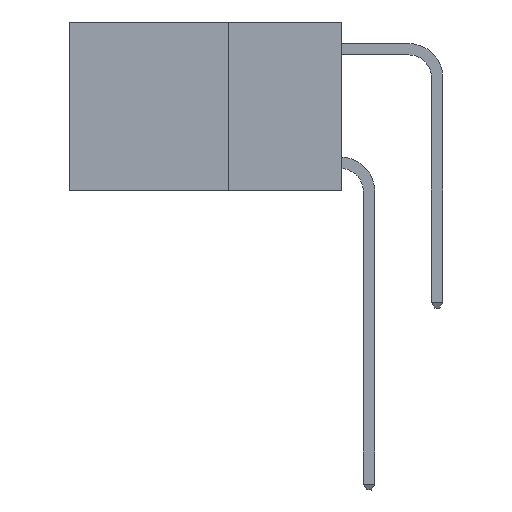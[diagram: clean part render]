
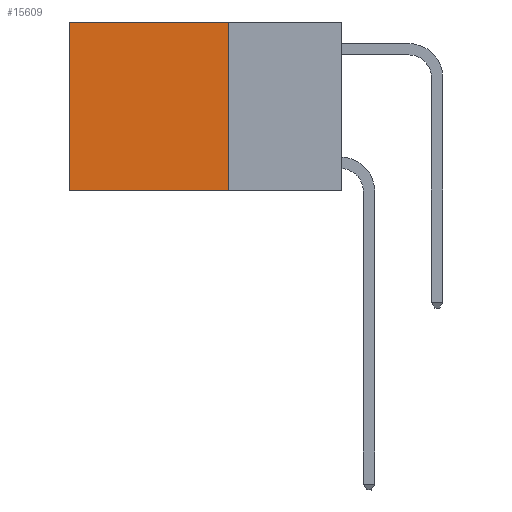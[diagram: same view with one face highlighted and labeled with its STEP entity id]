
A CAD part, left-side view. The second image highlights one B-rep face of the part: STEP entity #15609.
In plain terms, the highlighted planar face has unit normal (-1, 0, 0).
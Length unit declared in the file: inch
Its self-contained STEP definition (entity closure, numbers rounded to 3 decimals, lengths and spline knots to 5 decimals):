
#139 = DIRECTION ( 'NONE',  ( 0., 0., -1. ) ) ;
#140 = VERTEX_POINT ( 'NONE', #27110 ) ;
#480 = CARTESIAN_POINT ( 'NONE',  ( 0.2625, 0.25, -0.37 ) ) ;
#797 = LINE ( 'NONE', #14445, #27979 ) ;
#2272 = VERTEX_POINT ( 'NONE', #8109 ) ;
#2958 = ORIENTED_EDGE ( 'NONE', *, *, #20229, .F. ) ;
#4125 = CARTESIAN_POINT ( 'NONE',  ( 0.2625, 0.25, 0. ) ) ;
#4859 = DIRECTION ( 'NONE',  ( 1., 0., 0. ) ) ;
#5541 = ORIENTED_EDGE ( 'NONE', *, *, #27164, .T. ) ;
#6876 = CARTESIAN_POINT ( 'NONE',  ( 0.2625, 0.25, 0. ) ) ;
#8109 = CARTESIAN_POINT ( 'NONE',  ( 0.2625, 0.6, 0. ) ) ;
#8999 = VECTOR ( 'NONE', #139, 39.37008 ) ;
#10046 = LINE ( 'NONE', #480, #14059 ) ;
#11615 = ORIENTED_EDGE ( 'NONE', *, *, #28678, .T. ) ;
#11720 = DIRECTION ( 'NONE',  ( 0., 0., -1. ) ) ;
#12388 = ORIENTED_EDGE ( 'NONE', *, *, #13680, .F. ) ;
#13089 = LINE ( 'NONE', #4125, #23575 ) ;
#13672 = VERTEX_POINT ( 'NONE', #6876 ) ;
#13680 = EDGE_CURVE ( 'NONE', #13672, #140, #18396, .T. ) ;
#14059 = VECTOR ( 'NONE', #21457, 39.37008 ) ;
#14445 = CARTESIAN_POINT ( 'NONE',  ( 0.2625, 0.6, 0. ) ) ;
#15609 = ADVANCED_FACE ( 'NONE', ( #18771 ), #16224, .F. ) ;
#15784 = DIRECTION ( 'NONE',  ( 0., 1., 0. ) ) ;
#16224 = PLANE ( 'NONE',  #17961 ) ;
#16360 = EDGE_LOOP ( 'NONE', ( #11615, #2958, #12388, #5541 ) ) ;
#16820 = DIRECTION ( 'NONE',  ( 0., 0., -1. ) ) ;
#17961 = AXIS2_PLACEMENT_3D ( 'NONE', #25406, #4859, #11720 ) ;
#18396 = LINE ( 'NONE', #25043, #8999 ) ;
#18771 = FACE_OUTER_BOUND ( 'NONE', #16360, .T. ) ;
#20229 = EDGE_CURVE ( 'NONE', #140, #26815, #10046, .T. ) ;
#21457 = DIRECTION ( 'NONE',  ( 0., 1., 0. ) ) ;
#23575 = VECTOR ( 'NONE', #15784, 39.37008 ) ;
#25043 = CARTESIAN_POINT ( 'NONE',  ( 0.2625, 0.25, 0. ) ) ;
#25285 = CARTESIAN_POINT ( 'NONE',  ( 0.2625, 0.6, -0.37 ) ) ;
#25406 = CARTESIAN_POINT ( 'NONE',  ( 0.2625, 0.25, 0. ) ) ;
#26815 = VERTEX_POINT ( 'NONE', #25285 ) ;
#27110 = CARTESIAN_POINT ( 'NONE',  ( 0.2625, 0.25, -0.37 ) ) ;
#27164 = EDGE_CURVE ( 'NONE', #13672, #2272, #13089, .T. ) ;
#27979 = VECTOR ( 'NONE', #16820, 39.37008 ) ;
#28678 = EDGE_CURVE ( 'NONE', #2272, #26815, #797, .T. ) ;
